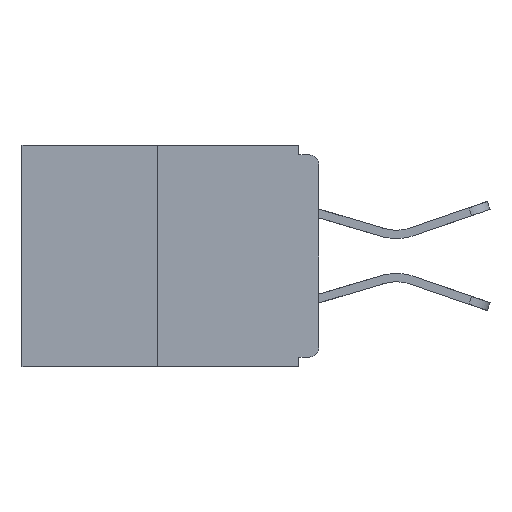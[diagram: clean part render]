
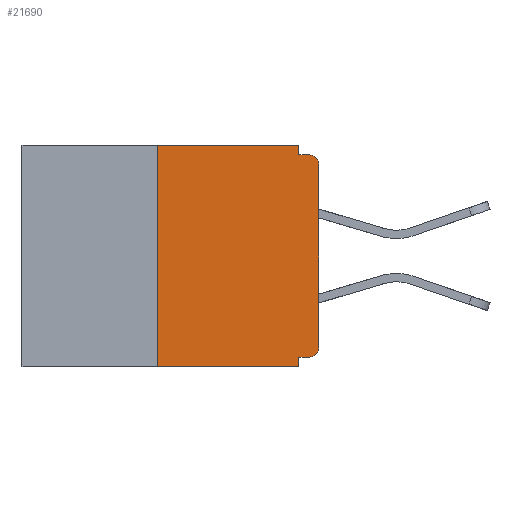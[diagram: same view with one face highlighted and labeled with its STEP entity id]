
A CAD part, left-side view. The second image highlights one B-rep face of the part: STEP entity #21690.
In plain terms, the highlighted planar face has unit normal (-1, 0, 0).
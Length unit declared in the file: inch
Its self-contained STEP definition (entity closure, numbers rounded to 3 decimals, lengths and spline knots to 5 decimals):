
#108 = DIRECTION ( 'NONE',  ( -1., 0., 0. ) ) ;
#275 = LINE ( 'NONE', #3763, #20907 ) ;
#971 = VECTOR ( 'NONE', #15773, 39.37008 ) ;
#1129 = ORIENTED_EDGE ( 'NONE', *, *, #12528, .F. ) ;
#1264 = CARTESIAN_POINT ( 'NONE',  ( 0., 0.031, 0. ) ) ;
#1737 = VERTEX_POINT ( 'NONE', #1264 ) ;
#2027 = ORIENTED_EDGE ( 'NONE', *, *, #18926, .T. ) ;
#2071 = LINE ( 'NONE', #10411, #17312 ) ;
#3001 = CARTESIAN_POINT ( 'NONE',  ( 0., 0., -0.313 ) ) ;
#3763 = CARTESIAN_POINT ( 'NONE',  ( 0., 0., 0. ) ) ;
#3893 = EDGE_LOOP ( 'NONE', ( #17007, #22158, #8003, #15777, #10206, #7450, #2027, #15646, #1129, #11383 ) ) ;
#3938 = EDGE_CURVE ( 'NONE', #13805, #19816, #24943, .T. ) ;
#4378 = CARTESIAN_POINT ( 'NONE',  ( 0., 0.031, 0. ) ) ;
#4466 = DIRECTION ( 'NONE',  ( 0., 0., -1. ) ) ;
#4680 = AXIS2_PLACEMENT_3D ( 'NONE', #23518, #5474, #15486 ) ;
#4886 = CARTESIAN_POINT ( 'NONE',  ( 0., 0.46, 0. ) ) ;
#5474 = DIRECTION ( 'NONE',  ( -1., 0., 0. ) ) ;
#5532 = LINE ( 'NONE', #12891, #22702 ) ;
#6138 = CARTESIAN_POINT ( 'NONE',  ( 0., 0., -0.328 ) ) ;
#6284 = LINE ( 'NONE', #20168, #21898 ) ;
#6785 = EDGE_CURVE ( 'NONE', #19213, #1737, #9782, .T. ) ;
#6894 = DIRECTION ( 'NONE',  ( 1., 0., 0. ) ) ;
#7245 = VERTEX_POINT ( 'NONE', #15048 ) ;
#7450 = ORIENTED_EDGE ( 'NONE', *, *, #8150, .T. ) ;
#7974 = DIRECTION ( 'NONE',  ( 0., 0., 1. ) ) ;
#8003 = ORIENTED_EDGE ( 'NONE', *, *, #16748, .T. ) ;
#8150 = EDGE_CURVE ( 'NONE', #24169, #17522, #14357, .T. ) ;
#8634 = EDGE_CURVE ( 'NONE', #24169, #20272, #10905, .T. ) ;
#8733 = VECTOR ( 'NONE', #25017, 39.37008 ) ;
#8833 = DIRECTION ( 'NONE',  ( 0., -1., 0. ) ) ;
#9402 = LINE ( 'NONE', #4378, #24781 ) ;
#9782 = LINE ( 'NONE', #13642, #971 ) ;
#10132 = CARTESIAN_POINT ( 'NONE',  ( 0., 0.031, -0.343 ) ) ;
#10206 = ORIENTED_EDGE ( 'NONE', *, *, #8634, .F. ) ;
#10411 = CARTESIAN_POINT ( 'NONE',  ( 0., 0.25, 0. ) ) ;
#10758 = PLANE ( 'NONE',  #25365 ) ;
#10905 = LINE ( 'NONE', #6138, #11235 ) ;
#11118 = CARTESIAN_POINT ( 'NONE',  ( 0., 0., -0.015 ) ) ;
#11235 = VECTOR ( 'NONE', #22098, 39.37008 ) ;
#11383 = ORIENTED_EDGE ( 'NONE', *, *, #24604, .F. ) ;
#12090 = CARTESIAN_POINT ( 'NONE',  ( 0., 0., -0.03 ) ) ;
#12266 = DIRECTION ( 'NONE',  ( 0., 0., 1. ) ) ;
#12528 = EDGE_CURVE ( 'NONE', #16571, #19816, #23708, .T. ) ;
#12891 = CARTESIAN_POINT ( 'NONE',  ( 0., 0.031, -0.343 ) ) ;
#13105 = VERTEX_POINT ( 'NONE', #10132 ) ;
#13642 = CARTESIAN_POINT ( 'NONE',  ( 0., 0.46, 0. ) ) ;
#13805 = VERTEX_POINT ( 'NONE', #12090 ) ;
#14357 = CIRCLE ( 'NONE', #4680, 0.015 ) ;
#14784 = CARTESIAN_POINT ( 'NONE',  ( 0., 0.25, 0. ) ) ;
#15048 = CARTESIAN_POINT ( 'NONE',  ( 0., 0.25, -0.343 ) ) ;
#15095 = CARTESIAN_POINT ( 'NONE',  ( 0., 0.031, -0.328 ) ) ;
#15486 = DIRECTION ( 'NONE',  ( 0., 0., -1. ) ) ;
#15646 = ORIENTED_EDGE ( 'NONE', *, *, #3938, .T. ) ;
#15773 = DIRECTION ( 'NONE',  ( 0., -1., 0. ) ) ;
#15777 = ORIENTED_EDGE ( 'NONE', *, *, #25676, .F. ) ;
#16571 = VERTEX_POINT ( 'NONE', #17119 ) ;
#16748 = EDGE_CURVE ( 'NONE', #7245, #13105, #6284, .T. ) ;
#16956 = CARTESIAN_POINT ( 'NONE',  ( 0., 0.015, -0.015 ) ) ;
#17007 = ORIENTED_EDGE ( 'NONE', *, *, #6785, .F. ) ;
#17119 = CARTESIAN_POINT ( 'NONE',  ( 0., 0.031, -0.015 ) ) ;
#17312 = VECTOR ( 'NONE', #12266, 39.37008 ) ;
#17522 = VERTEX_POINT ( 'NONE', #3001 ) ;
#18609 = CARTESIAN_POINT ( 'NONE',  ( 0., 0.015, -0.328 ) ) ;
#18926 = EDGE_CURVE ( 'NONE', #17522, #13805, #275, .T. ) ;
#19213 = VERTEX_POINT ( 'NONE', #14784 ) ;
#19505 = FACE_OUTER_BOUND ( 'NONE', #3893, .T. ) ;
#19816 = VERTEX_POINT ( 'NONE', #16956 ) ;
#20130 = CARTESIAN_POINT ( 'NONE',  ( 0., 0.015, -0.03 ) ) ;
#20168 = CARTESIAN_POINT ( 'NONE',  ( 0., 0.46, -0.343 ) ) ;
#20272 = VERTEX_POINT ( 'NONE', #15095 ) ;
#20296 = DIRECTION ( 'NONE',  ( 0., 0., -1. ) ) ;
#20833 = DIRECTION ( 'NONE',  ( 0., 0., -1. ) ) ;
#20907 = VECTOR ( 'NONE', #7974, 39.37008 ) ;
#21690 = ADVANCED_FACE ( 'NONE', ( #19505 ), #10758, .F. ) ;
#21875 = EDGE_CURVE ( 'NONE', #7245, #19213, #2071, .T. ) ;
#21898 = VECTOR ( 'NONE', #8833, 39.37008 ) ;
#22098 = DIRECTION ( 'NONE',  ( 0., 1., 0. ) ) ;
#22158 = ORIENTED_EDGE ( 'NONE', *, *, #21875, .F. ) ;
#22702 = VECTOR ( 'NONE', #22786, 39.37008 ) ;
#22786 = DIRECTION ( 'NONE',  ( 0., 0., -1. ) ) ;
#22807 = AXIS2_PLACEMENT_3D ( 'NONE', #20130, #108, #20296 ) ;
#23518 = CARTESIAN_POINT ( 'NONE',  ( 0., 0.015, -0.313 ) ) ;
#23708 = LINE ( 'NONE', #11118, #8733 ) ;
#24169 = VERTEX_POINT ( 'NONE', #18609 ) ;
#24604 = EDGE_CURVE ( 'NONE', #1737, #16571, #9402, .T. ) ;
#24781 = VECTOR ( 'NONE', #4466, 39.37008 ) ;
#24943 = CIRCLE ( 'NONE', #22807, 0.015 ) ;
#25017 = DIRECTION ( 'NONE',  ( 0., -1., 0. ) ) ;
#25365 = AXIS2_PLACEMENT_3D ( 'NONE', #4886, #6894, #20833 ) ;
#25676 = EDGE_CURVE ( 'NONE', #20272, #13105, #5532, .T. ) ;
